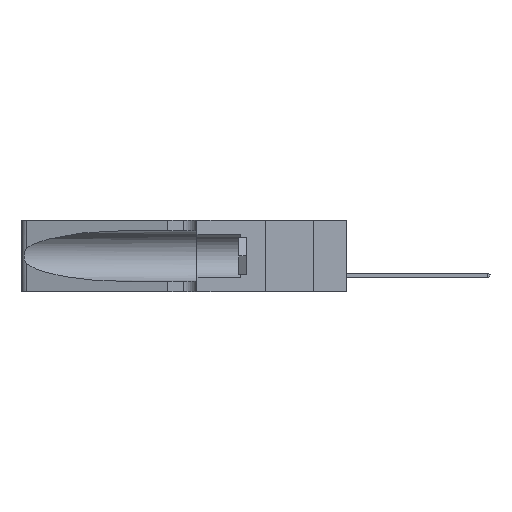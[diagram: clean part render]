
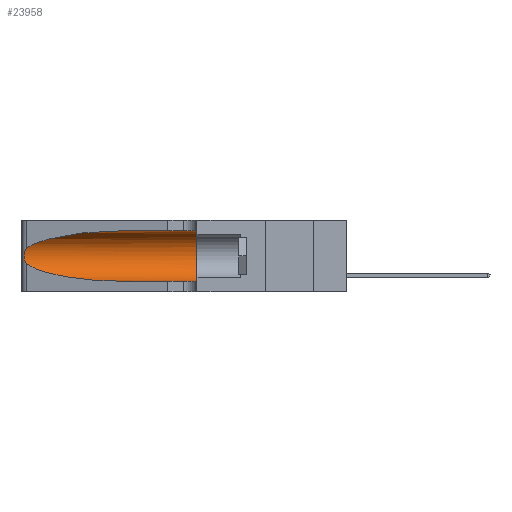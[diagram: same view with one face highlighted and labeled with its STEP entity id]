
A CAD part, left-side view. The second image highlights one B-rep face of the part: STEP entity #23958.
In plain terms, the highlighted cylindrical face has radius 3.308 mm (diameter 6.617 mm), a partial arc.
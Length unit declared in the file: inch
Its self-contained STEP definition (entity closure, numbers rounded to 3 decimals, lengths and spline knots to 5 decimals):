
#204 = CARTESIAN_POINT ( 'NONE',  ( 0.1305, 0.72297, 0.05475 ) ) ;
#628 = CARTESIAN_POINT ( 'NONE',  ( 0.2373, 1.15595, 0.08982 ) ) ;
#1463 = EDGE_CURVE ( 'NONE', #20552, #14174, #8175, .T. ) ;
#2487 = LINE ( 'NONE', #40118, #42224 ) ;
#2654 = CARTESIAN_POINT ( 'NONE',  ( 0.1305, 0.72297, 0.05475 ) ) ;
#3407 = CARTESIAN_POINT ( 'NONE',  ( 0.25555, 1.22994, 0.2215 ) ) ;
#3503 = ORIENTED_EDGE ( 'NONE', *, *, #10423, .F. ) ;
#3535 = VECTOR ( 'NONE', #26501, 39.37008 ) ;
#4088 = ORIENTED_EDGE ( 'NONE', *, *, #21436, .T. ) ;
#4752 = CARTESIAN_POINT ( 'NONE',  ( 0.2373, 1.15595, 0.28018 ) ) ;
#4790 = VERTEX_POINT ( 'NONE', #33779 ) ;
#4900 = CARTESIAN_POINT ( 'NONE',  ( 0.25639, 1.23186, 0.15144 ) ) ;
#6264 = CARTESIAN_POINT ( 'NONE',  ( 0.25487, 1.22718, 0.22369 ) ) ;
#6283 = EDGE_LOOP ( 'NONE', ( #33692, #4088, #20949, #11358, #16384, #3503 ) ) ;
#7097 = DIRECTION ( 'NONE',  ( 0., 0., 1. ) ) ;
#7236 = CARTESIAN_POINT ( 'NONE',  ( 0.1305, 0.35, 0.185 ) ) ;
#8175 =( BOUNDED_CURVE ( )  B_SPLINE_CURVE ( 3, ( #21532, #628, #14106, #204 ),
 .UNSPECIFIED., .F., .F. ) 
 B_SPLINE_CURVE_WITH_KNOTS ( ( 4, 4 ),
 ( 3.44316, 4.71239 ),
 .UNSPECIFIED. ) 
 CURVE ( )  GEOMETRIC_REPRESENTATION_ITEM ( )  RATIONAL_B_SPLINE_CURVE ( ( 1., 0.87, 0.87, 1. ) ) 
 REPRESENTATION_ITEM ( '' )  );
#10360 = CARTESIAN_POINT ( 'NONE',  ( 0.1305, 0.35, 0.05475 ) ) ;
#10423 = EDGE_CURVE ( 'NONE', #35332, #24867, #31394, .T. ) ;
#10916 = CARTESIAN_POINT ( 'NONE',  ( 0.1305, 0.72297, 0.31525 ) ) ;
#11358 = ORIENTED_EDGE ( 'NONE', *, *, #27890, .T. ) ;
#12426 = CARTESIAN_POINT ( 'NONE',  ( 0.26075, 1.23896, 0.178 ) ) ;
#13642 = VERTEX_POINT ( 'NONE', #10360 ) ;
#14106 = CARTESIAN_POINT ( 'NONE',  ( 0.18966, 0.96281, 0.05475 ) ) ;
#14174 = VERTEX_POINT ( 'NONE', #2654 ) ;
#14257 = EDGE_CURVE ( 'NONE', #35332, #4790, #37218, .T. ) ;
#15954 = CARTESIAN_POINT ( 'NONE',  ( 0.1305, 1.61858, 0.31525 ) ) ;
#16197 = CARTESIAN_POINT ( 'NONE',  ( 0.25555, 1.22993, 0.14849 ) ) ;
#16384 = ORIENTED_EDGE ( 'NONE', *, *, #41487, .F. ) ;
#17596 = CARTESIAN_POINT ( 'NONE',  ( 0.18966, 0.96281, 0.31525 ) ) ;
#17890 = CARTESIAN_POINT ( 'NONE',  ( 0.25487, 1.22718, 0.22369 ) ) ;
#18034 = CARTESIAN_POINT ( 'NONE',  ( 0.26018, 1.23835, 0.19895 ) ) ;
#18223 = B_SPLINE_CURVE_WITH_KNOTS ( 'NONE', 3,
 ( #17890, #3407, #36013, #18639, #22137, #18034, #26104, #12426, #26438, #32671, #22296, #4900, #16197, #36925 ),
 .UNSPECIFIED., .F., .F.,
 ( 4, 2, 2, 2, 2, 2, 4 ),
 ( 0., 0.00027, 0.00053, 0.00107, 0.0016, 0.00187, 0.00214 ),
 .UNSPECIFIED. ) ;
#18639 = CARTESIAN_POINT ( 'NONE',  ( 0.25787, 1.23484, 0.2124 ) ) ;
#19126 = CYLINDRICAL_SURFACE ( 'NONE', #44404, 0.13025 ) ;
#19707 = CARTESIAN_POINT ( 'NONE',  ( 0.1305, 0.35, 0.31525 ) ) ;
#20225 = FACE_OUTER_BOUND ( 'NONE', #6283, .T. ) ;
#20552 = VERTEX_POINT ( 'NONE', #38721 ) ;
#20949 = ORIENTED_EDGE ( 'NONE', *, *, #1463, .T. ) ;
#21130 = CARTESIAN_POINT ( 'NONE',  ( 0.1305, 1.61858, 0.185 ) ) ;
#21436 = EDGE_CURVE ( 'NONE', #4790, #20552, #18223, .T. ) ;
#21532 = CARTESIAN_POINT ( 'NONE',  ( 0.25487, 1.22718, 0.14631 ) ) ;
#22137 = CARTESIAN_POINT ( 'NONE',  ( 0.25854, 1.2359, 0.20912 ) ) ;
#22296 = CARTESIAN_POINT ( 'NONE',  ( 0.25789, 1.23486, 0.15765 ) ) ;
#23958 = ADVANCED_FACE ( 'NONE', ( #20225 ), #19126, .F. ) ;
#24630 = DIRECTION ( 'NONE',  ( 0., 0., -1. ) ) ;
#24786 = DIRECTION ( 'NONE',  ( 0., -1., 0. ) ) ;
#24867 = VERTEX_POINT ( 'NONE', #19707 ) ;
#26104 = CARTESIAN_POINT ( 'NONE',  ( 0.26075, 1.23896, 0.19203 ) ) ;
#26438 = CARTESIAN_POINT ( 'NONE',  ( 0.26017, 1.23833, 0.17102 ) ) ;
#26501 = DIRECTION ( 'NONE',  ( 0., -1., 0. ) ) ;
#27890 = EDGE_CURVE ( 'NONE', #14174, #13642, #2487, .T. ) ;
#27972 = DIRECTION ( 'NONE',  ( 0., 1., 0. ) ) ;
#28123 = CIRCLE ( 'NONE', #38081, 0.13025 ) ;
#31394 = LINE ( 'NONE', #15954, #3535 ) ;
#32671 = CARTESIAN_POINT ( 'NONE',  ( 0.25856, 1.23593, 0.16098 ) ) ;
#33692 = ORIENTED_EDGE ( 'NONE', *, *, #14257, .T. ) ;
#33779 = CARTESIAN_POINT ( 'NONE',  ( 0.25487, 1.22718, 0.22369 ) ) ;
#35332 = VERTEX_POINT ( 'NONE', #10916 ) ;
#36013 = CARTESIAN_POINT ( 'NONE',  ( 0.25639, 1.23184, 0.21858 ) ) ;
#36925 = CARTESIAN_POINT ( 'NONE',  ( 0.25487, 1.22718, 0.14631 ) ) ;
#37218 =( BOUNDED_CURVE ( )  B_SPLINE_CURVE ( 3, ( #42481, #17596, #4752, #6264 ),
 .UNSPECIFIED., .F., .T. ) 
 B_SPLINE_CURVE_WITH_KNOTS ( ( 4, 4 ),
 ( 1.5708, 2.84003 ),
 .UNSPECIFIED. ) 
 CURVE ( )  GEOMETRIC_REPRESENTATION_ITEM ( )  RATIONAL_B_SPLINE_CURVE ( ( 1., 0.87, 0.87, 1. ) ) 
 REPRESENTATION_ITEM ( '' )  );
#38081 = AXIS2_PLACEMENT_3D ( 'NONE', #7236, #27972, #7097 ) ;
#38721 = CARTESIAN_POINT ( 'NONE',  ( 0.25487, 1.22718, 0.14631 ) ) ;
#39810 = DIRECTION ( 'NONE',  ( 0., -1., 0. ) ) ;
#40118 = CARTESIAN_POINT ( 'NONE',  ( 0.1305, 1.61858, 0.05475 ) ) ;
#41487 = EDGE_CURVE ( 'NONE', #24867, #13642, #28123, .T. ) ;
#42224 = VECTOR ( 'NONE', #39810, 39.37008 ) ;
#42481 = CARTESIAN_POINT ( 'NONE',  ( 0.1305, 0.72297, 0.31525 ) ) ;
#44404 = AXIS2_PLACEMENT_3D ( 'NONE', #21130, #24786, #24630 ) ;
